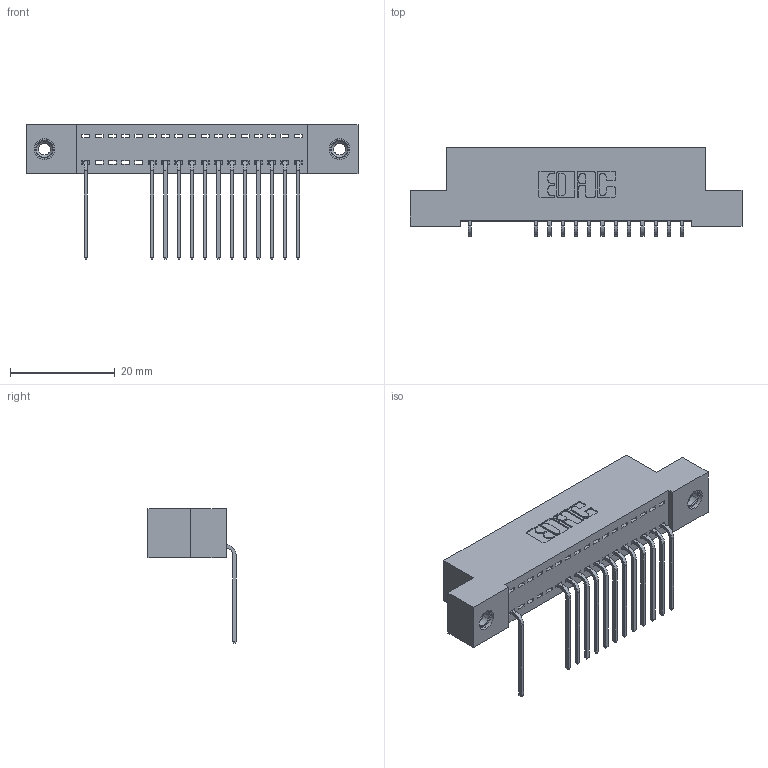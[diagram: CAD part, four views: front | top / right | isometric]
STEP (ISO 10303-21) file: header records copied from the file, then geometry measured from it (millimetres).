
FILE_DESCRIPTION (( 'STEP AP203' ), '1' );
FILE_NAME ('392-017-559-108.STEP', '2018-08-15T03:28:25', ( '' ), ( '' ), 'SwSTEP 2.0', 'SolidWorks 2016', '' );
FILE_SCHEMA (( 'CONFIG_CONTROL_DESIGN' ));
Length unit declared in the file: inch
Products named in the file (4): 345-292-001_558 559 Tail - 1; 345-250-001_345-250-003-102; 392-017-559-108; 342 Part_TI
Assembly tree (16 placements, depth 2):
  392-017-559-108
    342 Part_TI
    345-292-001_558 559 Tail - 1  x13
    345-250-001_345-250-003-102  x2
Bounding box: 63.5 x 16.83 x 25.78 mm (x, y, z)
Volume: 5467.5 mm3; surface area: 7588.7 mm2
Topology: 16 solids, 16 shells, 998 faces, 2969 edges, 1954 vertices
Faces by surface type: plane 718, cylinder 264, cone 12, torus 4
Entity records: 14636 total; most frequent: CARTESIAN_POINT 2528, ORIENTED_EDGE 2478, DIRECTION 2211, EDGE_CURVE 1239, VECTOR 1091, LINE 1091, VERTEX_POINT 820, AXIS2_PLACEMENT_3D 560
